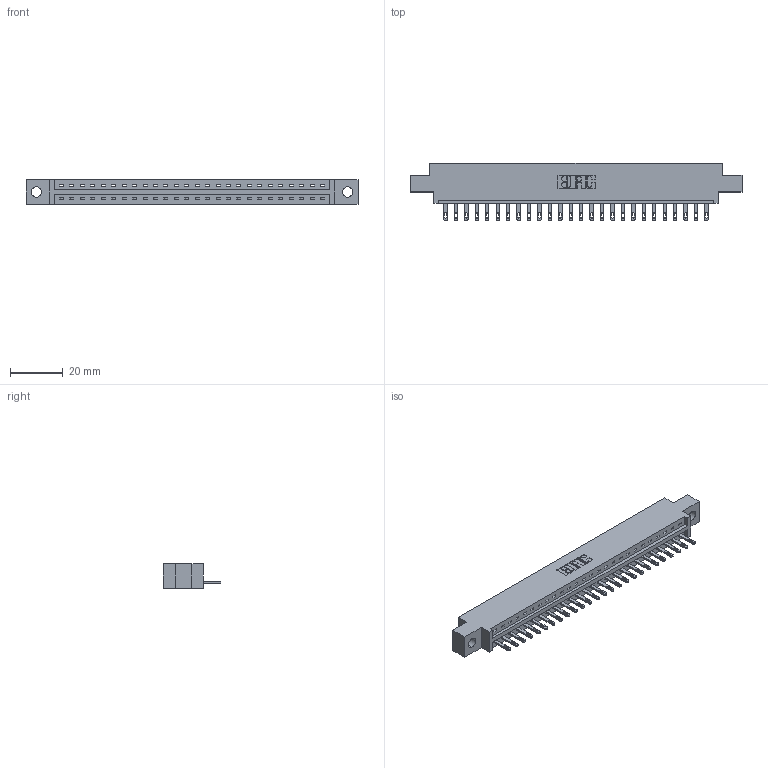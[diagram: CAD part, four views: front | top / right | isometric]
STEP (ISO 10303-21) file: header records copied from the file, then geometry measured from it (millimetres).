
FILE_DESCRIPTION (( 'STEP AP203' ), '1' );
FILE_NAME ('887-026-500-604.STEP', '2020-09-20T19:39:17', ( '' ), ( '' ), 'SwSTEP 2.0', 'SolidWorks 2020', '' );
FILE_SCHEMA (( 'CONFIG_CONTROL_DESIGN' ));
Length unit declared in the file: inch
Products named in the file (3): 887-026-500-604; 837 Part_0.170 Offset - 0.156 Dia-TH; 345-292-001_345-293-100
Assembly tree (27 placements, depth 2):
  887-026-500-604
    837 Part_0.170 Offset - 0.156 Dia-TH
    345-292-001_345-293-100  x26
Bounding box: 126.03 x 21.85 x 9.4 mm (x, y, z)
Volume: 12709.7 mm3; surface area: 12997.2 mm2
Topology: 27 solids, 27 shells, 1626 faces, 5003 edges, 3334 vertices
Faces by surface type: plane 1114, cylinder 512
Entity records: 21461 total; most frequent: CARTESIAN_POINT 3744, ORIENTED_EDGE 3706, DIRECTION 3185, EDGE_CURVE 1853, VECTOR 1721, LINE 1721, VERTEX_POINT 1234, AXIS2_PLACEMENT_3D 732
